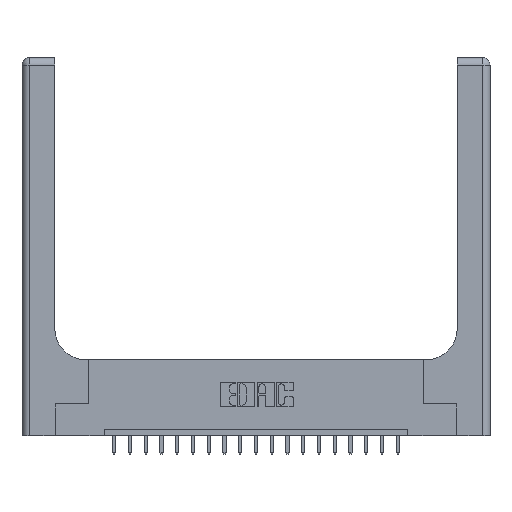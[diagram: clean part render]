
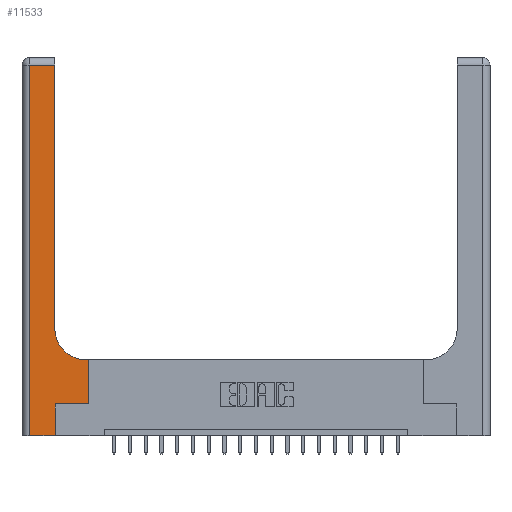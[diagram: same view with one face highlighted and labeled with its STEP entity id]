
A CAD part, top view. The second image highlights one B-rep face of the part: STEP entity #11533.
In plain terms, the highlighted planar face has unit normal (0, 0, 1).
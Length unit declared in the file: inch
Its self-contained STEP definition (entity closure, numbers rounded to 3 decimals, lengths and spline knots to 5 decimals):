
#213 = DIRECTION ( 'NONE',  ( -1., 0., 0. ) ) ;
#421 = VERTEX_POINT ( 'NONE', #18477 ) ;
#562 = DIRECTION ( 'NONE',  ( 1., 0., 0. ) ) ;
#635 = VECTOR ( 'NONE', #11812, 39.37008 ) ;
#976 = CARTESIAN_POINT ( 'NONE',  ( 0.265, 0., 0.37 ) ) ;
#996 = AXIS2_PLACEMENT_3D ( 'NONE', #10589, #5875, #11993 ) ;
#1294 = ORIENTED_EDGE ( 'NONE', *, *, #5923, .T. ) ;
#2420 = VERTEX_POINT ( 'NONE', #12861 ) ;
#2657 = VERTEX_POINT ( 'NONE', #5968 ) ;
#2869 = CARTESIAN_POINT ( 'NONE',  ( 0., 2.94, 0.37 ) ) ;
#3058 = VERTEX_POINT ( 'NONE', #10637 ) ;
#3075 = EDGE_CURVE ( 'NONE', #10010, #16344, #13759, .T. ) ;
#3407 = VERTEX_POINT ( 'NONE', #12124 ) ;
#3510 = ORIENTED_EDGE ( 'NONE', *, *, #5672, .T. ) ;
#3537 = VERTEX_POINT ( 'NONE', #8157 ) ;
#3811 = VECTOR ( 'NONE', #9981, 39.37008 ) ;
#3845 = VECTOR ( 'NONE', #17004, 39.37008 ) ;
#4805 = LINE ( 'NONE', #18925, #14536 ) ;
#4967 = CARTESIAN_POINT ( 'NONE',  ( 0.528, 0.6, 0.37 ) ) ;
#5229 = ORIENTED_EDGE ( 'NONE', *, *, #6904, .T. ) ;
#5672 = EDGE_CURVE ( 'NONE', #3058, #3407, #15280, .T. ) ;
#5875 = DIRECTION ( 'NONE',  ( 0., 0., -1. ) ) ;
#5923 = EDGE_CURVE ( 'NONE', #13008, #2420, #4805, .T. ) ;
#5928 = VECTOR ( 'NONE', #562, 39.37008 ) ;
#5968 = CARTESIAN_POINT ( 'NONE',  ( 0.265, 0.25, 0.37 ) ) ;
#6521 = LINE ( 'NONE', #9801, #14105 ) ;
#6642 = EDGE_CURVE ( 'NONE', #2420, #421, #18865, .T. ) ;
#6711 = DIRECTION ( 'NONE',  ( 1., 0., 0. ) ) ;
#6904 = EDGE_CURVE ( 'NONE', #16344, #2657, #8896, .T. ) ;
#7732 = ORIENTED_EDGE ( 'NONE', *, *, #12241, .T. ) ;
#8116 = ORIENTED_EDGE ( 'NONE', *, *, #6642, .T. ) ;
#8157 = CARTESIAN_POINT ( 'NONE',  ( 0.528, 0.25, 0.37 ) ) ;
#8534 = ORIENTED_EDGE ( 'NONE', *, *, #10985, .T. ) ;
#8871 = PLANE ( 'NONE',  #996 ) ;
#8896 = LINE ( 'NONE', #976, #635 ) ;
#8987 = ORIENTED_EDGE ( 'NONE', *, *, #17732, .T. ) ;
#9498 = CARTESIAN_POINT ( 'NONE',  ( 0., 0., 0.37 ) ) ;
#9565 = ORIENTED_EDGE ( 'NONE', *, *, #3075, .T. ) ;
#9801 = CARTESIAN_POINT ( 'NONE',  ( 0.265, 0.25, 0.37 ) ) ;
#9892 = CARTESIAN_POINT ( 'NONE',  ( 0.06, 3., 0.37 ) ) ;
#9981 = DIRECTION ( 'NONE',  ( 0., 1., 0. ) ) ;
#10010 = VERTEX_POINT ( 'NONE', #12864 ) ;
#10589 = CARTESIAN_POINT ( 'NONE',  ( 0., 3., 0.37 ) ) ;
#10637 = CARTESIAN_POINT ( 'NONE',  ( 0.26, 2.94, 0.37 ) ) ;
#10754 = DIRECTION ( 'NONE',  ( 0., 1., 0. ) ) ;
#10985 = EDGE_CURVE ( 'NONE', #3407, #10010, #11640, .T. ) ;
#11246 = CARTESIAN_POINT ( 'NONE',  ( 0.265, 0., 0.37 ) ) ;
#11458 = CARTESIAN_POINT ( 'NONE',  ( 0.26, 3., 0.37 ) ) ;
#11533 = ADVANCED_FACE ( 'NONE', ( #13844 ), #8871, .F. ) ;
#11640 = LINE ( 'NONE', #9892, #12636 ) ;
#11812 = DIRECTION ( 'NONE',  ( 0., 1., 0. ) ) ;
#11993 = DIRECTION ( 'NONE',  ( -1., 0., 0. ) ) ;
#12124 = CARTESIAN_POINT ( 'NONE',  ( 0.06, 2.94, 0.37 ) ) ;
#12241 = EDGE_CURVE ( 'NONE', #421, #3058, #12561, .T. ) ;
#12354 = DIRECTION ( 'NONE',  ( 0., 0., -1. ) ) ;
#12561 = LINE ( 'NONE', #11458, #3811 ) ;
#12630 = LINE ( 'NONE', #16919, #13888 ) ;
#12636 = VECTOR ( 'NONE', #18950, 39.37008 ) ;
#12861 = CARTESIAN_POINT ( 'NONE',  ( 0.51, 0.6, 0.37 ) ) ;
#12864 = CARTESIAN_POINT ( 'NONE',  ( 0.06, 0., 0.37 ) ) ;
#13008 = VERTEX_POINT ( 'NONE', #4967 ) ;
#13759 = LINE ( 'NONE', #9498, #5928 ) ;
#13844 = FACE_OUTER_BOUND ( 'NONE', #19651, .T. ) ;
#13888 = VECTOR ( 'NONE', #10754, 39.37008 ) ;
#13946 = DIRECTION ( 'NONE',  ( 1., 0., 0. ) ) ;
#14105 = VECTOR ( 'NONE', #6711, 39.37008 ) ;
#14536 = VECTOR ( 'NONE', #213, 39.37008 ) ;
#15280 = LINE ( 'NONE', #2869, #3845 ) ;
#16344 = VERTEX_POINT ( 'NONE', #11246 ) ;
#16879 = ORIENTED_EDGE ( 'NONE', *, *, #18345, .T. ) ;
#16919 = CARTESIAN_POINT ( 'NONE',  ( 0.528, 0.25, 0.37 ) ) ;
#17004 = DIRECTION ( 'NONE',  ( -1., 0., 0. ) ) ;
#17732 = EDGE_CURVE ( 'NONE', #2657, #3537, #6521, .T. ) ;
#18071 = AXIS2_PLACEMENT_3D ( 'NONE', #19978, #12354, #13946 ) ;
#18345 = EDGE_CURVE ( 'NONE', #3537, #13008, #12630, .T. ) ;
#18477 = CARTESIAN_POINT ( 'NONE',  ( 0.26, 0.85, 0.37 ) ) ;
#18865 = CIRCLE ( 'NONE', #18071, 0.25 ) ;
#18925 = CARTESIAN_POINT ( 'NONE',  ( 0.26, 0.6, 0.37 ) ) ;
#18950 = DIRECTION ( 'NONE',  ( 0., -1., 0. ) ) ;
#19651 = EDGE_LOOP ( 'NONE', ( #7732, #3510, #8534, #9565, #5229, #8987, #16879, #1294, #8116 ) ) ;
#19978 = CARTESIAN_POINT ( 'NONE',  ( 0.51, 0.85, 0.37 ) ) ;
